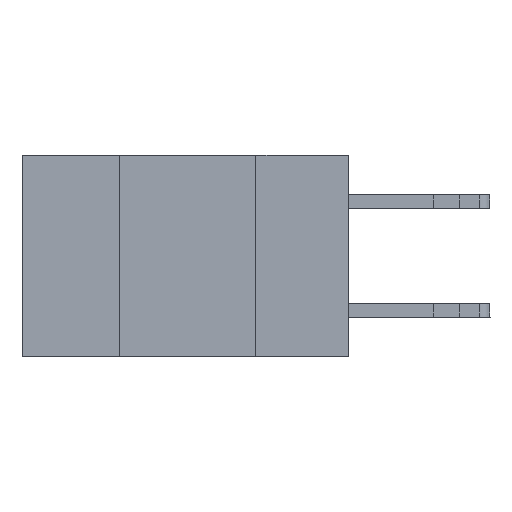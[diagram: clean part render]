
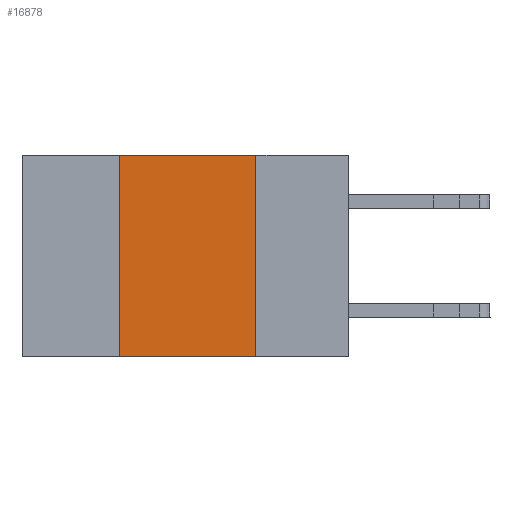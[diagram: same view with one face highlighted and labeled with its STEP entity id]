
A CAD part, left-side view. The second image highlights one B-rep face of the part: STEP entity #16878.
In plain terms, the highlighted planar face has unit normal (-1, 0, 0).
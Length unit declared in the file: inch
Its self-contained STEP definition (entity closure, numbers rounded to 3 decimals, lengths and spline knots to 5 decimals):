
#412 = CARTESIAN_POINT ( 'NONE',  ( 0., 0.42, 0. ) ) ;
#981 = FACE_OUTER_BOUND ( 'NONE', #5193, .T. ) ;
#1434 = CARTESIAN_POINT ( 'NONE',  ( 0., 0.6, -0.37 ) ) ;
#1546 = CARTESIAN_POINT ( 'NONE',  ( 0., 0.6, 0. ) ) ;
#2821 = CARTESIAN_POINT ( 'NONE',  ( 0., 0.17, 0. ) ) ;
#3925 = EDGE_CURVE ( 'NONE', #18689, #19462, #15141, .T. ) ;
#4868 = ORIENTED_EDGE ( 'NONE', *, *, #10673, .F. ) ;
#5026 = LINE ( 'NONE', #412, #14642 ) ;
#5193 = EDGE_LOOP ( 'NONE', ( #4868, #10345, #20036, #12075 ) ) ;
#6120 = CARTESIAN_POINT ( 'NONE',  ( 0., 0.6, 0. ) ) ;
#7093 = DIRECTION ( 'NONE',  ( 0., 0., 1. ) ) ;
#7284 = VERTEX_POINT ( 'NONE', #11457 ) ;
#8026 = CARTESIAN_POINT ( 'NONE',  ( 0., 0.42, -0.37 ) ) ;
#10179 = VECTOR ( 'NONE', #15949, 39.37008 ) ;
#10187 = VECTOR ( 'NONE', #18803, 39.37008 ) ;
#10345 = ORIENTED_EDGE ( 'NONE', *, *, #16777, .F. ) ;
#10673 = EDGE_CURVE ( 'NONE', #17066, #19462, #14407, .T. ) ;
#11150 = PLANE ( 'NONE',  #17397 ) ;
#11218 = DIRECTION ( 'NONE',  ( 0., 0., -1. ) ) ;
#11457 = CARTESIAN_POINT ( 'NONE',  ( 0., 0.42, 0. ) ) ;
#12075 = ORIENTED_EDGE ( 'NONE', *, *, #3925, .T. ) ;
#14012 = CARTESIAN_POINT ( 'NONE',  ( 0., 0.17, 0. ) ) ;
#14070 = EDGE_CURVE ( 'NONE', #18689, #7284, #5026, .T. ) ;
#14334 = DIRECTION ( 'NONE',  ( 1., 0., 0. ) ) ;
#14407 = LINE ( 'NONE', #2821, #10179 ) ;
#14642 = VECTOR ( 'NONE', #7093, 39.37008 ) ;
#15141 = LINE ( 'NONE', #1434, #10187 ) ;
#15435 = DIRECTION ( 'NONE',  ( 0., -1., 0. ) ) ;
#15949 = DIRECTION ( 'NONE',  ( 0., 0., -1. ) ) ;
#16777 = EDGE_CURVE ( 'NONE', #7284, #17066, #18986, .T. ) ;
#16878 = ADVANCED_FACE ( 'NONE', ( #981 ), #11150, .F. ) ;
#17066 = VERTEX_POINT ( 'NONE', #14012 ) ;
#17263 = VECTOR ( 'NONE', #15435, 39.37008 ) ;
#17397 = AXIS2_PLACEMENT_3D ( 'NONE', #1546, #14334, #11218 ) ;
#18689 = VERTEX_POINT ( 'NONE', #8026 ) ;
#18803 = DIRECTION ( 'NONE',  ( 0., -1., 0. ) ) ;
#18986 = LINE ( 'NONE', #6120, #17263 ) ;
#19130 = CARTESIAN_POINT ( 'NONE',  ( 0., 0.17, -0.37 ) ) ;
#19462 = VERTEX_POINT ( 'NONE', #19130 ) ;
#20036 = ORIENTED_EDGE ( 'NONE', *, *, #14070, .F. ) ;
